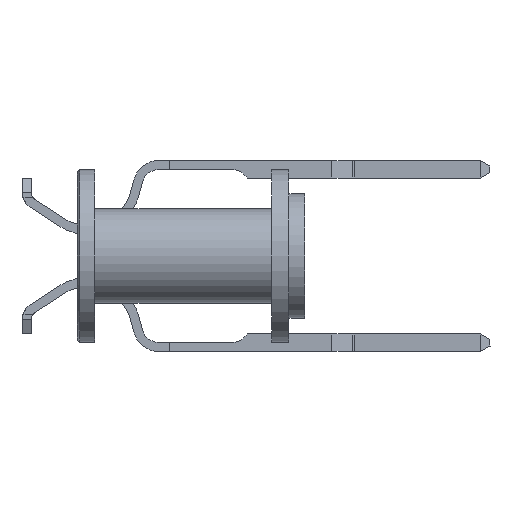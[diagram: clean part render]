
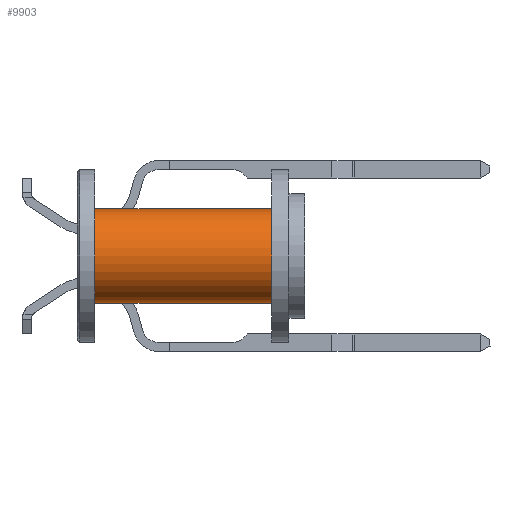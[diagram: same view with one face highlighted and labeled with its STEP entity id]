
A CAD part, left-side view. The second image highlights one B-rep face of the part: STEP entity #9903.
In plain terms, the highlighted cylindrical face has radius 1.727 mm (diameter 3.454 mm), a partial arc.
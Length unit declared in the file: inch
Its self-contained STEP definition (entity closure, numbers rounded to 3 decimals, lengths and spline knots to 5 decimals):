
#590 = EDGE_LOOP ( 'NONE', ( #18677, #18149, #24156, #25963 ) ) ;
#995 = CYLINDRICAL_SURFACE ( 'NONE', #24498, 0.068 ) ;
#5098 = EDGE_CURVE ( 'NONE', #9123, #8023, #25717, .T. ) ;
#5633 = DIRECTION ( 'NONE',  ( 0., 1., 0. ) ) ;
#5967 = CARTESIAN_POINT ( 'NONE',  ( 0., 0.025, -0.068 ) ) ;
#6174 = CARTESIAN_POINT ( 'NONE',  ( 0., 0.28, 0. ) ) ;
#7327 = LINE ( 'NONE', #11263, #18138 ) ;
#7417 = EDGE_CURVE ( 'NONE', #10921, #9123, #13325, .T. ) ;
#7482 = DIRECTION ( 'NONE',  ( 0., 0., -1. ) ) ;
#8023 = VERTEX_POINT ( 'NONE', #5967 ) ;
#8123 = AXIS2_PLACEMENT_3D ( 'NONE', #18513, #5633, #20607 ) ;
#8347 = DIRECTION ( 'NONE',  ( 0., 0., 1. ) ) ;
#9123 = VERTEX_POINT ( 'NONE', #16260 ) ;
#9903 = ADVANCED_FACE ( 'NONE', ( #23865 ), #995, .T. ) ;
#10456 = CARTESIAN_POINT ( 'NONE',  ( 0., 0.28, -0.068 ) ) ;
#10921 = VERTEX_POINT ( 'NONE', #15255 ) ;
#11263 = CARTESIAN_POINT ( 'NONE',  ( 0., 0.328, -0.068 ) ) ;
#12680 = DIRECTION ( 'NONE',  ( 0., -1., 0. ) ) ;
#13325 = LINE ( 'NONE', #25386, #18376 ) ;
#13739 = VERTEX_POINT ( 'NONE', #10456 ) ;
#13880 = CARTESIAN_POINT ( 'NONE',  ( 0., 0.328, 0. ) ) ;
#15255 = CARTESIAN_POINT ( 'NONE',  ( 0., 0.28, 0.068 ) ) ;
#16260 = CARTESIAN_POINT ( 'NONE',  ( 0., 0.025, 0.068 ) ) ;
#16413 = AXIS2_PLACEMENT_3D ( 'NONE', #6174, #21146, #8347 ) ;
#18138 = VECTOR ( 'NONE', #24039, 39.37008 ) ;
#18149 = ORIENTED_EDGE ( 'NONE', *, *, #7417, .T. ) ;
#18376 = VECTOR ( 'NONE', #12680, 39.37008 ) ;
#18513 = CARTESIAN_POINT ( 'NONE',  ( 0., 0.025, 0. ) ) ;
#18677 = ORIENTED_EDGE ( 'NONE', *, *, #24797, .F. ) ;
#18882 = CIRCLE ( 'NONE', #16413, 0.068 ) ;
#20001 = EDGE_CURVE ( 'NONE', #13739, #8023, #7327, .T. ) ;
#20304 = DIRECTION ( 'NONE',  ( 0., -1., 0. ) ) ;
#20607 = DIRECTION ( 'NONE',  ( 0., 0., 1. ) ) ;
#21146 = DIRECTION ( 'NONE',  ( 0., 1., 0. ) ) ;
#23865 = FACE_OUTER_BOUND ( 'NONE', #590, .T. ) ;
#24039 = DIRECTION ( 'NONE',  ( 0., -1., 0. ) ) ;
#24156 = ORIENTED_EDGE ( 'NONE', *, *, #5098, .T. ) ;
#24498 = AXIS2_PLACEMENT_3D ( 'NONE', #13880, #20304, #7482 ) ;
#24797 = EDGE_CURVE ( 'NONE', #10921, #13739, #18882, .T. ) ;
#25386 = CARTESIAN_POINT ( 'NONE',  ( 0., 0.328, 0.068 ) ) ;
#25717 = CIRCLE ( 'NONE', #8123, 0.068 ) ;
#25963 = ORIENTED_EDGE ( 'NONE', *, *, #20001, .F. ) ;
